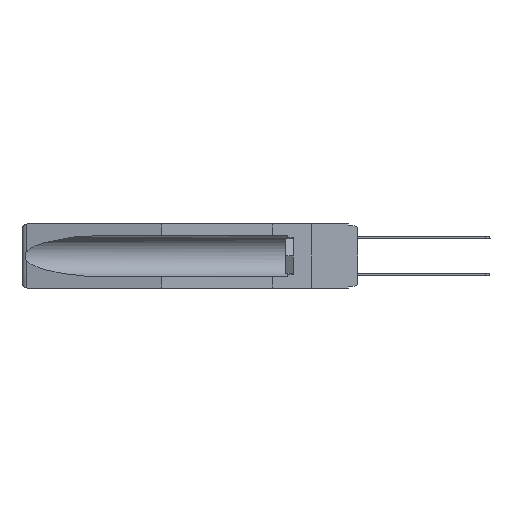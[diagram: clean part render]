
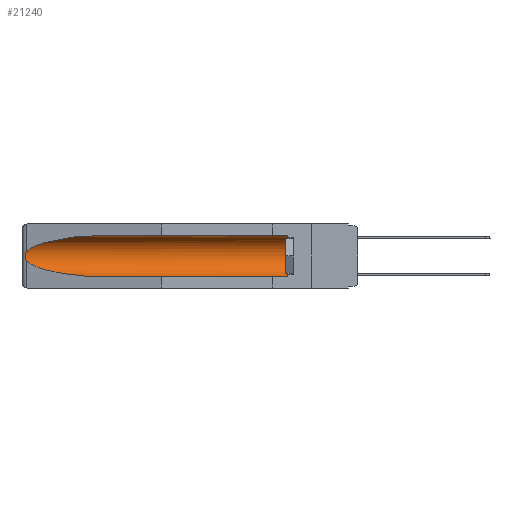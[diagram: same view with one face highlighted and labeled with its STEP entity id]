
A CAD part, left-side view. The second image highlights one B-rep face of the part: STEP entity #21240.
In plain terms, the highlighted cylindrical face has radius 2.857 mm (diameter 5.715 mm), a partial arc.
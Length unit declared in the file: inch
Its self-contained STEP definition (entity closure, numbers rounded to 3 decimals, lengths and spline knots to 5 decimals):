
#60 = CARTESIAN_POINT ( 'NONE',  ( 0.2673, 1.53269, -0.17917 ) ) ;
#432 = AXIS2_PLACEMENT_3D ( 'NONE', #13537, #16878, #18557 ) ;
#546 = LINE ( 'NONE', #17181, #17069 ) ;
#907 = EDGE_CURVE ( 'NONE', #11210, #4496, #13957, .T. ) ;
#1116 = CARTESIAN_POINT ( 'NONE',  ( 0.26537, 1.52718, -0.19328 ) ) ;
#1236 = EDGE_CURVE ( 'NONE', #7220, #4496, #546, .T. ) ;
#1387 = CARTESIAN_POINT ( 'NONE',  ( 0.155, 0.126, -0.059 ) ) ;
#1432 = CARTESIAN_POINT ( 'NONE',  ( 0.26537, 1.52718, -0.19328 ) ) ;
#1502 = AXIS2_PLACEMENT_3D ( 'NONE', #6840, #3534, #15086 ) ;
#1709 = ORIENTED_EDGE ( 'NONE', *, *, #2368, .T. ) ;
#1757 = CARTESIAN_POINT ( 'NONE',  ( 0.26537, 1.52718, -0.19328 ) ) ;
#2368 = EDGE_CURVE ( 'NONE', #7220, #18305, #5152, .T. ) ;
#2420 = ORIENTED_EDGE ( 'NONE', *, *, #8909, .T. ) ;
#3470 = CARTESIAN_POINT ( 'NONE',  ( 0.155, 0.126, -0.284 ) ) ;
#3534 = DIRECTION ( 'NONE',  ( 0., -1., 0. ) ) ;
#3570 = LINE ( 'NONE', #7562, #7959 ) ;
#4453 = CARTESIAN_POINT ( 'NONE',  ( 0.26537, 1.52718, -0.14972 ) ) ;
#4496 = VERTEX_POINT ( 'NONE', #9634 ) ;
#5152 = CIRCLE ( 'NONE', #1502, 0.1125 ) ;
#5770 = DIRECTION ( 'NONE',  ( 0., 1., 0. ) ) ;
#6121 = DIRECTION ( 'NONE',  ( 0., 1., 0. ) ) ;
#6580 = CARTESIAN_POINT ( 'NONE',  ( 0.26654, 1.53092, -0.15636 ) ) ;
#6686 = CARTESIAN_POINT ( 'NONE',  ( 0.155, 1.07973, -0.284 ) ) ;
#6840 = CARTESIAN_POINT ( 'NONE',  ( 0.155, 0.126, -0.1715 ) ) ;
#7220 = VERTEX_POINT ( 'NONE', #3470 ) ;
#7562 = CARTESIAN_POINT ( 'NONE',  ( 0.155, -0.30754, -0.059 ) ) ;
#7931 = EDGE_LOOP ( 'NONE', ( #14958, #2420, #9042, #17220, #1709, #18447 ) ) ;
#7959 = VECTOR ( 'NONE', #6121, 39.37008 ) ;
#8232 = CARTESIAN_POINT ( 'NONE',  ( 0.26655, 1.53094, -0.18657 ) ) ;
#8909 = EDGE_CURVE ( 'NONE', #13350, #11210, #10899, .T. ) ;
#9042 = ORIENTED_EDGE ( 'NONE', *, *, #907, .T. ) ;
#9439 = CARTESIAN_POINT ( 'NONE',  ( 0.155, 1.07973, -0.059 ) ) ;
#9634 = CARTESIAN_POINT ( 'NONE',  ( 0.155, 1.07973, -0.284 ) ) ;
#9931 = CARTESIAN_POINT ( 'NONE',  ( 0.21114, 1.30732, -0.284 ) ) ;
#10899 = B_SPLINE_CURVE_WITH_KNOTS ( 'NONE', 3,
 ( #16424, #13296, #6580, #11690, #11617, #19833, #60, #8232, #18168, #1757 ),
 .UNSPECIFIED., .F., .F.,
 ( 4, 2, 2, 2, 4 ),
 ( 0., 0.00029, 0.00058, 0.00087, 0.00117 ),
 .UNSPECIFIED. ) ;
#11210 = VERTEX_POINT ( 'NONE', #1116 ) ;
#11585 = CARTESIAN_POINT ( 'NONE',  ( 0.26537, 1.52718, -0.14972 ) ) ;
#11617 = CARTESIAN_POINT ( 'NONE',  ( 0.2675, 1.53308, -0.16763 ) ) ;
#11690 = CARTESIAN_POINT ( 'NONE',  ( 0.2673, 1.5327, -0.16383 ) ) ;
#13136 =( BOUNDED_CURVE ( )  B_SPLINE_CURVE ( 3, ( #9439, #21187, #16247, #11585 ),
 .UNSPECIFIED., .F., .F. ) 
 B_SPLINE_CURVE_WITH_KNOTS ( ( 4, 4 ),
 ( 4.71239, 6.08839 ),
 .UNSPECIFIED. ) 
 CURVE ( )  GEOMETRIC_REPRESENTATION_ITEM ( )  RATIONAL_B_SPLINE_CURVE ( ( 1., 0.848, 0.848, 1. ) ) 
 REPRESENTATION_ITEM ( '' )  );
#13296 = CARTESIAN_POINT ( 'NONE',  ( 0.26597, 1.52961, -0.15275 ) ) ;
#13350 = VERTEX_POINT ( 'NONE', #4453 ) ;
#13537 = CARTESIAN_POINT ( 'NONE',  ( 0.155, -0.30754, -0.1715 ) ) ;
#13957 =( BOUNDED_CURVE ( )  B_SPLINE_CURVE ( 3, ( #1432, #21255, #9931, #6686 ),
 .UNSPECIFIED., .F., .F. ) 
 B_SPLINE_CURVE_WITH_KNOTS ( ( 4, 4 ),
 ( 0.1948, 1.5708 ),
 .UNSPECIFIED. ) 
 CURVE ( )  GEOMETRIC_REPRESENTATION_ITEM ( )  RATIONAL_B_SPLINE_CURVE ( ( 1., 0.848, 0.848, 1. ) ) 
 REPRESENTATION_ITEM ( '' )  );
#14958 = ORIENTED_EDGE ( 'NONE', *, *, #16705, .T. ) ;
#15086 = DIRECTION ( 'NONE',  ( 0., 0., 1. ) ) ;
#15662 = CYLINDRICAL_SURFACE ( 'NONE', #432, 0.1125 ) ;
#16247 = CARTESIAN_POINT ( 'NONE',  ( 0.25451, 1.48313, -0.09465 ) ) ;
#16424 = CARTESIAN_POINT ( 'NONE',  ( 0.26537, 1.52718, -0.14972 ) ) ;
#16705 = EDGE_CURVE ( 'NONE', #21010, #13350, #13136, .T. ) ;
#16878 = DIRECTION ( 'NONE',  ( 0., 1., 0. ) ) ;
#17026 = CARTESIAN_POINT ( 'NONE',  ( 0.155, 1.07973, -0.059 ) ) ;
#17069 = VECTOR ( 'NONE', #5770, 39.37008 ) ;
#17171 = EDGE_CURVE ( 'NONE', #18305, #21010, #3570, .T. ) ;
#17181 = CARTESIAN_POINT ( 'NONE',  ( 0.155, -0.30754, -0.284 ) ) ;
#17220 = ORIENTED_EDGE ( 'NONE', *, *, #1236, .F. ) ;
#18168 = CARTESIAN_POINT ( 'NONE',  ( 0.26597, 1.5296, -0.19026 ) ) ;
#18305 = VERTEX_POINT ( 'NONE', #1387 ) ;
#18447 = ORIENTED_EDGE ( 'NONE', *, *, #17171, .T. ) ;
#18557 = DIRECTION ( 'NONE',  ( 0., 0., 1. ) ) ;
#19548 = FACE_OUTER_BOUND ( 'NONE', #7931, .T. ) ;
#19833 = CARTESIAN_POINT ( 'NONE',  ( 0.2675, 1.53308, -0.17534 ) ) ;
#21010 = VERTEX_POINT ( 'NONE', #17026 ) ;
#21187 = CARTESIAN_POINT ( 'NONE',  ( 0.21114, 1.30732, -0.059 ) ) ;
#21240 = ADVANCED_FACE ( 'NONE', ( #19548 ), #15662, .F. ) ;
#21255 = CARTESIAN_POINT ( 'NONE',  ( 0.25451, 1.48313, -0.24835 ) ) ;
